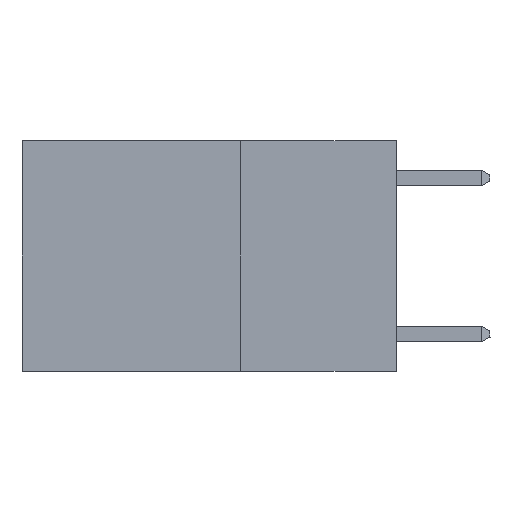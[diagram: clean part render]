
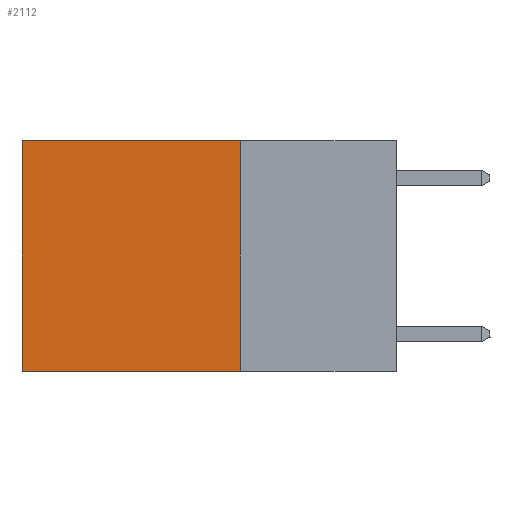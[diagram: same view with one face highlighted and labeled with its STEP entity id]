
A CAD part, left-side view. The second image highlights one B-rep face of the part: STEP entity #2112.
In plain terms, the highlighted planar face has unit normal (-1, 0, 0).
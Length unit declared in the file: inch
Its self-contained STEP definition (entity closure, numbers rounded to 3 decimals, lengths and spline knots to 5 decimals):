
#947 = CARTESIAN_POINT ( 'NONE',  ( 0.2625, 0.25, 0. ) ) ;
#1489 = DIRECTION ( 'NONE',  ( 0., 0., -1. ) ) ;
#2112 = ADVANCED_FACE ( 'NONE', ( #9785 ), #24594, .F. ) ;
#2831 = VERTEX_POINT ( 'NONE', #7337 ) ;
#3262 = EDGE_CURVE ( 'NONE', #12507, #2831, #14589, .T. ) ;
#5596 = LINE ( 'NONE', #7372, #24859 ) ;
#6155 = VERTEX_POINT ( 'NONE', #20010 ) ;
#6508 = CARTESIAN_POINT ( 'NONE',  ( 0.2625, 0.25, -0.37 ) ) ;
#7337 = CARTESIAN_POINT ( 'NONE',  ( 0.2625, 0.25, -0.37 ) ) ;
#7372 = CARTESIAN_POINT ( 'NONE',  ( 0.2625, 0.6, 0. ) ) ;
#8825 = CARTESIAN_POINT ( 'NONE',  ( 0.2625, 0.25, 0. ) ) ;
#9001 = LINE ( 'NONE', #8825, #23762 ) ;
#9313 = EDGE_CURVE ( 'NONE', #18505, #6155, #5596, .T. ) ;
#9785 = FACE_OUTER_BOUND ( 'NONE', #24477, .T. ) ;
#10043 = VECTOR ( 'NONE', #10433, 39.37008 ) ;
#10433 = DIRECTION ( 'NONE',  ( 0., 0., -1. ) ) ;
#11254 = DIRECTION ( 'NONE',  ( 0., 0., -1. ) ) ;
#12507 = VERTEX_POINT ( 'NONE', #947 ) ;
#13100 = DIRECTION ( 'NONE',  ( 1., 0., 0. ) ) ;
#13459 = ORIENTED_EDGE ( 'NONE', *, *, #9313, .T. ) ;
#13860 = EDGE_CURVE ( 'NONE', #12507, #18505, #9001, .T. ) ;
#14294 = DIRECTION ( 'NONE',  ( 0., 1., 0. ) ) ;
#14589 = LINE ( 'NONE', #21993, #10043 ) ;
#14704 = DIRECTION ( 'NONE',  ( 0., 1., 0. ) ) ;
#15143 = EDGE_CURVE ( 'NONE', #2831, #6155, #18345, .T. ) ;
#16555 = VECTOR ( 'NONE', #14294, 39.37008 ) ;
#16956 = CARTESIAN_POINT ( 'NONE',  ( 0.2625, 0.25, 0. ) ) ;
#18345 = LINE ( 'NONE', #6508, #16555 ) ;
#18446 = ORIENTED_EDGE ( 'NONE', *, *, #13860, .T. ) ;
#18505 = VERTEX_POINT ( 'NONE', #19161 ) ;
#19161 = CARTESIAN_POINT ( 'NONE',  ( 0.2625, 0.6, 0. ) ) ;
#19912 = AXIS2_PLACEMENT_3D ( 'NONE', #16956, #13100, #1489 ) ;
#20010 = CARTESIAN_POINT ( 'NONE',  ( 0.2625, 0.6, -0.37 ) ) ;
#21993 = CARTESIAN_POINT ( 'NONE',  ( 0.2625, 0.25, 0. ) ) ;
#23762 = VECTOR ( 'NONE', #14704, 39.37008 ) ;
#23795 = ORIENTED_EDGE ( 'NONE', *, *, #15143, .F. ) ;
#24018 = ORIENTED_EDGE ( 'NONE', *, *, #3262, .F. ) ;
#24477 = EDGE_LOOP ( 'NONE', ( #13459, #23795, #24018, #18446 ) ) ;
#24594 = PLANE ( 'NONE',  #19912 ) ;
#24859 = VECTOR ( 'NONE', #11254, 39.37008 ) ;
